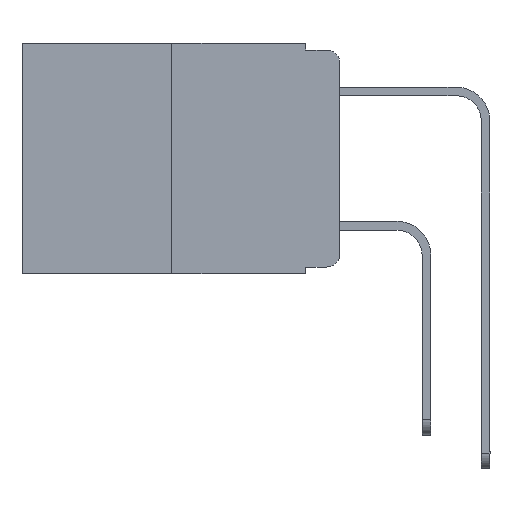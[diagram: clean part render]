
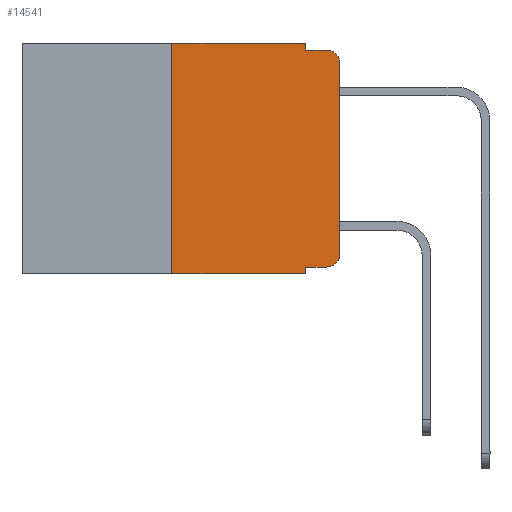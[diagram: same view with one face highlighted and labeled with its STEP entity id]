
A CAD part, left-side view. The second image highlights one B-rep face of the part: STEP entity #14541.
In plain terms, the highlighted planar face has unit normal (-1, 0, 0).
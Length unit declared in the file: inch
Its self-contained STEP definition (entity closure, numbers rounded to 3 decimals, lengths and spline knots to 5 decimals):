
#43 = DIRECTION ( 'NONE',  ( 1., 0., 0. ) ) ;
#151 = VERTEX_POINT ( 'NONE', #590 ) ;
#203 = EDGE_CURVE ( 'NONE', #5727, #9007, #7969, .T. ) ;
#221 = EDGE_CURVE ( 'NONE', #7975, #5727, #8817, .T. ) ;
#590 = CARTESIAN_POINT ( 'NONE',  ( 0., 0.25, 0. ) ) ;
#811 = DIRECTION ( 'NONE',  ( -1., 0., 0. ) ) ;
#925 = CARTESIAN_POINT ( 'NONE',  ( 0., 0.473, -0.343 ) ) ;
#991 = CIRCLE ( 'NONE', #11726, 0.02 ) ;
#1108 = DIRECTION ( 'NONE',  ( 0., -1., 0. ) ) ;
#1143 = DIRECTION ( 'NONE',  ( 0., 0., -1. ) ) ;
#1526 = EDGE_LOOP ( 'NONE', ( #8755, #6294, #3896, #12983, #10022, #3677, #12269, #4545, #12210, #4227 ) ) ;
#1613 = CARTESIAN_POINT ( 'NONE',  ( 0., 0.02, -0.03 ) ) ;
#2010 = EDGE_CURVE ( 'NONE', #7975, #3965, #12278, .T. ) ;
#2069 = CARTESIAN_POINT ( 'NONE',  ( 0., 0.051, 0. ) ) ;
#2188 = CARTESIAN_POINT ( 'NONE',  ( 0., 0.051, -0.01 ) ) ;
#2268 = PLANE ( 'NONE',  #5460 ) ;
#2562 = LINE ( 'NONE', #9299, #10680 ) ;
#2588 = DIRECTION ( 'NONE',  ( 0., 0., -1. ) ) ;
#2632 = CARTESIAN_POINT ( 'NONE',  ( 0., 0.02, -0.01 ) ) ;
#2901 = DIRECTION ( 'NONE',  ( 0., 0., 1. ) ) ;
#2908 = CARTESIAN_POINT ( 'NONE',  ( 0., 0.051, 0. ) ) ;
#3060 = CARTESIAN_POINT ( 'NONE',  ( 0., 0., -0.03 ) ) ;
#3117 = VERTEX_POINT ( 'NONE', #2908 ) ;
#3233 = CARTESIAN_POINT ( 'NONE',  ( 0., 0.25, -0.343 ) ) ;
#3439 = AXIS2_PLACEMENT_3D ( 'NONE', #6430, #811, #5315 ) ;
#3471 = DIRECTION ( 'NONE',  ( 0., 0., -1. ) ) ;
#3677 = ORIENTED_EDGE ( 'NONE', *, *, #14720, .F. ) ;
#3758 = DIRECTION ( 'NONE',  ( 0., 0., 1. ) ) ;
#3896 = ORIENTED_EDGE ( 'NONE', *, *, #4418, .F. ) ;
#3965 = VERTEX_POINT ( 'NONE', #6631 ) ;
#4069 = CARTESIAN_POINT ( 'NONE',  ( 0., 0.25, 0. ) ) ;
#4227 = ORIENTED_EDGE ( 'NONE', *, *, #203, .T. ) ;
#4359 = CARTESIAN_POINT ( 'NONE',  ( 0., 0., -0.313 ) ) ;
#4418 = EDGE_CURVE ( 'NONE', #6141, #10405, #6891, .T. ) ;
#4486 = LINE ( 'NONE', #12586, #10242 ) ;
#4545 = ORIENTED_EDGE ( 'NONE', *, *, #2010, .F. ) ;
#4878 = EDGE_CURVE ( 'NONE', #151, #3117, #4486, .T. ) ;
#5315 = DIRECTION ( 'NONE',  ( 0., 0., -1. ) ) ;
#5428 = CARTESIAN_POINT ( 'NONE',  ( 0., 0.02, -0.333 ) ) ;
#5460 = AXIS2_PLACEMENT_3D ( 'NONE', #9087, #43, #1143 ) ;
#5505 = DIRECTION ( 'NONE',  ( 0., -1., 0. ) ) ;
#5727 = VERTEX_POINT ( 'NONE', #5428 ) ;
#5808 = EDGE_CURVE ( 'NONE', #7357, #3965, #11142, .T. ) ;
#6141 = VERTEX_POINT ( 'NONE', #2188 ) ;
#6294 = ORIENTED_EDGE ( 'NONE', *, *, #9502, .T. ) ;
#6430 = CARTESIAN_POINT ( 'NONE',  ( 0., 0.02, -0.313 ) ) ;
#6631 = CARTESIAN_POINT ( 'NONE',  ( 0., 0.051, -0.343 ) ) ;
#6887 = EDGE_CURVE ( 'NONE', #9007, #12085, #9910, .T. ) ;
#6891 = LINE ( 'NONE', #10256, #14100 ) ;
#7357 = VERTEX_POINT ( 'NONE', #3233 ) ;
#7969 = CIRCLE ( 'NONE', #3439, 0.02 ) ;
#7975 = VERTEX_POINT ( 'NONE', #8673 ) ;
#8673 = CARTESIAN_POINT ( 'NONE',  ( 0., 0.051, -0.333 ) ) ;
#8755 = ORIENTED_EDGE ( 'NONE', *, *, #6887, .T. ) ;
#8791 = VECTOR ( 'NONE', #3758, 39.37008 ) ;
#8817 = LINE ( 'NONE', #14670, #9163 ) ;
#9007 = VERTEX_POINT ( 'NONE', #4359 ) ;
#9087 = CARTESIAN_POINT ( 'NONE',  ( 0., 0.473, 0. ) ) ;
#9163 = VECTOR ( 'NONE', #10957, 39.37008 ) ;
#9299 = CARTESIAN_POINT ( 'NONE',  ( 0., 0.051, 0. ) ) ;
#9502 = EDGE_CURVE ( 'NONE', #12085, #10405, #991, .T. ) ;
#9910 = LINE ( 'NONE', #11076, #10473 ) ;
#10022 = ORIENTED_EDGE ( 'NONE', *, *, #4878, .F. ) ;
#10242 = VECTOR ( 'NONE', #1108, 39.37008 ) ;
#10256 = CARTESIAN_POINT ( 'NONE',  ( 0., 0.051, -0.01 ) ) ;
#10405 = VERTEX_POINT ( 'NONE', #2632 ) ;
#10473 = VECTOR ( 'NONE', #2901, 39.37008 ) ;
#10680 = VECTOR ( 'NONE', #3471, 39.37008 ) ;
#10957 = DIRECTION ( 'NONE',  ( 0., -1., 0. ) ) ;
#11076 = CARTESIAN_POINT ( 'NONE',  ( 0., 0., 0. ) ) ;
#11142 = LINE ( 'NONE', #925, #12143 ) ;
#11389 = DIRECTION ( 'NONE',  ( 0., 0., -1. ) ) ;
#11675 = VECTOR ( 'NONE', #11389, 39.37008 ) ;
#11726 = AXIS2_PLACEMENT_3D ( 'NONE', #1613, #13986, #2588 ) ;
#12085 = VERTEX_POINT ( 'NONE', #3060 ) ;
#12143 = VECTOR ( 'NONE', #5505, 39.37008 ) ;
#12210 = ORIENTED_EDGE ( 'NONE', *, *, #221, .T. ) ;
#12269 = ORIENTED_EDGE ( 'NONE', *, *, #5808, .T. ) ;
#12278 = LINE ( 'NONE', #2069, #11675 ) ;
#12586 = CARTESIAN_POINT ( 'NONE',  ( 0., 0.473, 0. ) ) ;
#12983 = ORIENTED_EDGE ( 'NONE', *, *, #14433, .F. ) ;
#13581 = DIRECTION ( 'NONE',  ( 0., -1., 0. ) ) ;
#13737 = FACE_OUTER_BOUND ( 'NONE', #1526, .T. ) ;
#13986 = DIRECTION ( 'NONE',  ( -1., 0., 0. ) ) ;
#14100 = VECTOR ( 'NONE', #13581, 39.37008 ) ;
#14261 = LINE ( 'NONE', #4069, #8791 ) ;
#14433 = EDGE_CURVE ( 'NONE', #3117, #6141, #2562, .T. ) ;
#14541 = ADVANCED_FACE ( 'NONE', ( #13737 ), #2268, .F. ) ;
#14670 = CARTESIAN_POINT ( 'NONE',  ( 0., 0.051, -0.333 ) ) ;
#14720 = EDGE_CURVE ( 'NONE', #7357, #151, #14261, .T. ) ;
